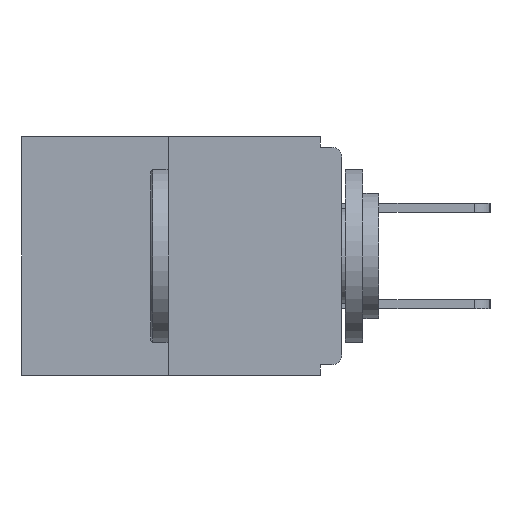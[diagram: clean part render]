
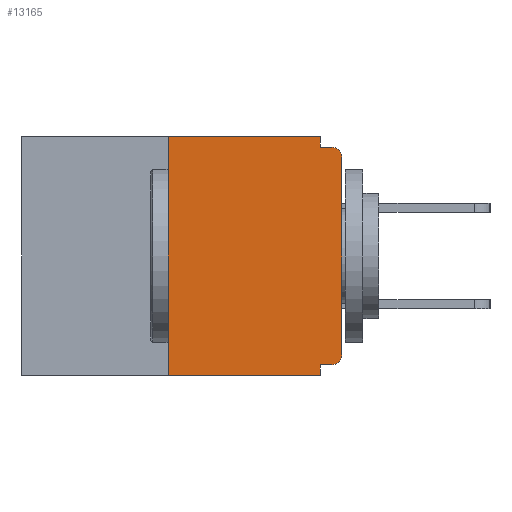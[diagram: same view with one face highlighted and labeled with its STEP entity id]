
A CAD part, left-side view. The second image highlights one B-rep face of the part: STEP entity #13165.
In plain terms, the highlighted planar face has unit normal (-1, 0, 0).
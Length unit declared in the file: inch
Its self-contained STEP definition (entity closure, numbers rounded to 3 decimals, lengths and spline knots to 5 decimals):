
#57 = EDGE_CURVE ( 'NONE', #19061, #18547, #12577, .T. ) ;
#165 = VERTEX_POINT ( 'NONE', #15347 ) ;
#249 = ORIENTED_EDGE ( 'NONE', *, *, #5438, .T. ) ;
#268 = DIRECTION ( 'NONE',  ( 1., 0., 0. ) ) ;
#419 = DIRECTION ( 'NONE',  ( 0., 0., -1. ) ) ;
#1103 = LINE ( 'NONE', #12187, #5233 ) ;
#1115 = ORIENTED_EDGE ( 'NONE', *, *, #14556, .F. ) ;
#1265 = VERTEX_POINT ( 'NONE', #10296 ) ;
#1605 = VECTOR ( 'NONE', #24027, 39.37008 ) ;
#2015 = ORIENTED_EDGE ( 'NONE', *, *, #15452, .F. ) ;
#2356 = DIRECTION ( 'NONE',  ( -1., 0., 0. ) ) ;
#2410 = CARTESIAN_POINT ( 'NONE',  ( 0., 0.46, -0.343 ) ) ;
#2529 = EDGE_LOOP ( 'NONE', ( #24108, #11616, #8043, #2015, #1115, #249, #16094, #7936, #5153, #23141 ) ) ;
#3038 = DIRECTION ( 'NONE',  ( 0., 0., -1. ) ) ;
#3377 = CARTESIAN_POINT ( 'NONE',  ( 0., 0.46, 0. ) ) ;
#3468 = DIRECTION ( 'NONE',  ( 0., -1., 0. ) ) ;
#4032 = CARTESIAN_POINT ( 'NONE',  ( 0., 0.25, 0. ) ) ;
#4129 = VECTOR ( 'NONE', #7457, 39.37008 ) ;
#4130 = CARTESIAN_POINT ( 'NONE',  ( 0., 0.46, 0. ) ) ;
#4653 = DIRECTION ( 'NONE',  ( 0., -1., 0. ) ) ;
#4862 = VECTOR ( 'NONE', #17837, 39.37008 ) ;
#5153 = ORIENTED_EDGE ( 'NONE', *, *, #8814, .F. ) ;
#5221 = CIRCLE ( 'NONE', #7386, 0.015 ) ;
#5233 = VECTOR ( 'NONE', #4653, 39.37008 ) ;
#5438 = EDGE_CURVE ( 'NONE', #23929, #165, #5221, .T. ) ;
#5591 = AXIS2_PLACEMENT_3D ( 'NONE', #12717, #5663, #7406 ) ;
#5663 = DIRECTION ( 'NONE',  ( -1., 0., 0. ) ) ;
#5857 = DIRECTION ( 'NONE',  ( 0., 0., 1. ) ) ;
#5960 = CARTESIAN_POINT ( 'NONE',  ( 0., 0.031, -0.015 ) ) ;
#7386 = AXIS2_PLACEMENT_3D ( 'NONE', #7798, #2356, #21227 ) ;
#7406 = DIRECTION ( 'NONE',  ( 0., 0., -1. ) ) ;
#7423 = VERTEX_POINT ( 'NONE', #19664 ) ;
#7457 = DIRECTION ( 'NONE',  ( 0., 0., 1. ) ) ;
#7798 = CARTESIAN_POINT ( 'NONE',  ( 0., 0.015, -0.313 ) ) ;
#7925 = CIRCLE ( 'NONE', #5591, 0.015 ) ;
#7936 = ORIENTED_EDGE ( 'NONE', *, *, #18269, .T. ) ;
#8043 = ORIENTED_EDGE ( 'NONE', *, *, #13784, .T. ) ;
#8814 = EDGE_CURVE ( 'NONE', #11161, #14027, #1103, .T. ) ;
#8869 = CARTESIAN_POINT ( 'NONE',  ( 0., 0.031, 0. ) ) ;
#9551 = PLANE ( 'NONE',  #15991 ) ;
#9619 = LINE ( 'NONE', #22629, #23392 ) ;
#10296 = CARTESIAN_POINT ( 'NONE',  ( 0., 0., -0.03 ) ) ;
#11161 = VERTEX_POINT ( 'NONE', #5960 ) ;
#11290 = LINE ( 'NONE', #22042, #1605 ) ;
#11616 = ORIENTED_EDGE ( 'NONE', *, *, #20004, .F. ) ;
#11833 = CARTESIAN_POINT ( 'NONE',  ( 0., 0.25, -0.343 ) ) ;
#11881 = CARTESIAN_POINT ( 'NONE',  ( 0., 0.25, 0. ) ) ;
#12007 = VECTOR ( 'NONE', #3468, 39.37008 ) ;
#12147 = CARTESIAN_POINT ( 'NONE',  ( 0., 0.031, 0. ) ) ;
#12187 = CARTESIAN_POINT ( 'NONE',  ( 0., 0., -0.015 ) ) ;
#12212 = LINE ( 'NONE', #2410, #4862 ) ;
#12577 = LINE ( 'NONE', #3377, #12007 ) ;
#12717 = CARTESIAN_POINT ( 'NONE',  ( 0., 0.015, -0.03 ) ) ;
#13165 = ADVANCED_FACE ( 'NONE', ( #20474 ), #9551, .F. ) ;
#13206 = VECTOR ( 'NONE', #3038, 39.37008 ) ;
#13651 = CARTESIAN_POINT ( 'NONE',  ( 0., 0.031, -0.343 ) ) ;
#13784 = EDGE_CURVE ( 'NONE', #15997, #22014, #12212, .T. ) ;
#14027 = VERTEX_POINT ( 'NONE', #18631 ) ;
#14556 = EDGE_CURVE ( 'NONE', #23929, #7423, #11290, .T. ) ;
#14985 = CARTESIAN_POINT ( 'NONE',  ( 0., 0., 0. ) ) ;
#15347 = CARTESIAN_POINT ( 'NONE',  ( 0., 0., -0.313 ) ) ;
#15452 = EDGE_CURVE ( 'NONE', #7423, #22014, #9619, .T. ) ;
#15716 = VECTOR ( 'NONE', #5857, 39.37008 ) ;
#15991 = AXIS2_PLACEMENT_3D ( 'NONE', #4130, #268, #419 ) ;
#15997 = VERTEX_POINT ( 'NONE', #11833 ) ;
#16094 = ORIENTED_EDGE ( 'NONE', *, *, #23043, .T. ) ;
#17550 = DIRECTION ( 'NONE',  ( 0., 0., -1. ) ) ;
#17837 = DIRECTION ( 'NONE',  ( 0., -1., 0. ) ) ;
#18053 = EDGE_CURVE ( 'NONE', #18547, #11161, #19383, .T. ) ;
#18269 = EDGE_CURVE ( 'NONE', #1265, #14027, #7925, .T. ) ;
#18547 = VERTEX_POINT ( 'NONE', #8869 ) ;
#18631 = CARTESIAN_POINT ( 'NONE',  ( 0., 0.015, -0.015 ) ) ;
#19061 = VERTEX_POINT ( 'NONE', #11881 ) ;
#19383 = LINE ( 'NONE', #12147, #13206 ) ;
#19664 = CARTESIAN_POINT ( 'NONE',  ( 0., 0.031, -0.328 ) ) ;
#20004 = EDGE_CURVE ( 'NONE', #15997, #19061, #23359, .T. ) ;
#20474 = FACE_OUTER_BOUND ( 'NONE', #2529, .T. ) ;
#20872 = LINE ( 'NONE', #14985, #4129 ) ;
#21227 = DIRECTION ( 'NONE',  ( 0., 0., -1. ) ) ;
#22014 = VERTEX_POINT ( 'NONE', #13651 ) ;
#22042 = CARTESIAN_POINT ( 'NONE',  ( 0., 0., -0.328 ) ) ;
#22629 = CARTESIAN_POINT ( 'NONE',  ( 0., 0.031, -0.343 ) ) ;
#22994 = CARTESIAN_POINT ( 'NONE',  ( 0., 0.015, -0.328 ) ) ;
#23043 = EDGE_CURVE ( 'NONE', #165, #1265, #20872, .T. ) ;
#23141 = ORIENTED_EDGE ( 'NONE', *, *, #18053, .F. ) ;
#23359 = LINE ( 'NONE', #4032, #15716 ) ;
#23392 = VECTOR ( 'NONE', #17550, 39.37008 ) ;
#23929 = VERTEX_POINT ( 'NONE', #22994 ) ;
#24027 = DIRECTION ( 'NONE',  ( 0., 1., 0. ) ) ;
#24108 = ORIENTED_EDGE ( 'NONE', *, *, #57, .F. ) ;
